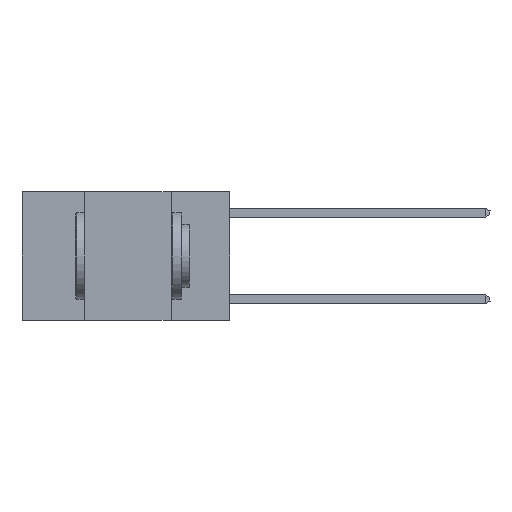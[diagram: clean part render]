
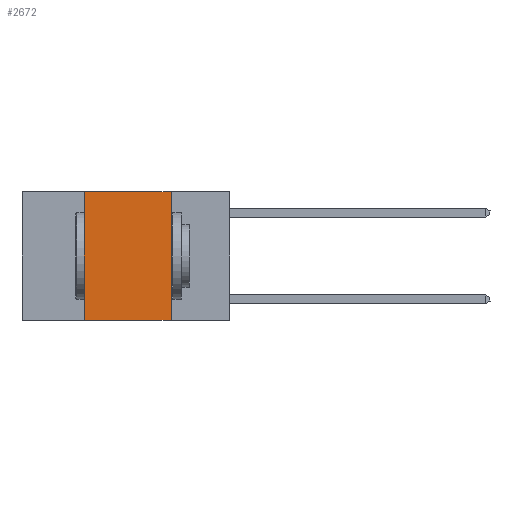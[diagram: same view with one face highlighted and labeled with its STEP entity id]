
A CAD part, left-side view. The second image highlights one B-rep face of the part: STEP entity #2672.
In plain terms, the highlighted planar face has unit normal (-1, 0, 0).
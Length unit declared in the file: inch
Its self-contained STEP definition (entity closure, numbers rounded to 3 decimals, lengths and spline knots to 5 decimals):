
#22 = CARTESIAN_POINT ( 'NONE',  ( 0., 0.6, 0. ) ) ;
#589 = EDGE_LOOP ( 'NONE', ( #2381, #4205, #6792, #6455 ) ) ;
#1487 = CARTESIAN_POINT ( 'NONE',  ( 0., 0.6, -0.37 ) ) ;
#2381 = ORIENTED_EDGE ( 'NONE', *, *, #10137, .F. ) ;
#2543 = CARTESIAN_POINT ( 'NONE',  ( 0., 0.42, 0. ) ) ;
#2587 = EDGE_CURVE ( 'NONE', #9000, #4918, #8205, .T. ) ;
#2672 = ADVANCED_FACE ( 'NONE', ( #7817 ), #2712, .F. ) ;
#2712 = PLANE ( 'NONE',  #8276 ) ;
#3847 = LINE ( 'NONE', #4020, #10657 ) ;
#3904 = VERTEX_POINT ( 'NONE', #10523 ) ;
#3906 = DIRECTION ( 'NONE',  ( 0., 0., -1. ) ) ;
#3972 = CARTESIAN_POINT ( 'NONE',  ( 0., 0.42, 0. ) ) ;
#4020 = CARTESIAN_POINT ( 'NONE',  ( 0., 0.17, 0. ) ) ;
#4205 = ORIENTED_EDGE ( 'NONE', *, *, #8605, .F. ) ;
#4883 = DIRECTION ( 'NONE',  ( 0., -1., 0. ) ) ;
#4918 = VERTEX_POINT ( 'NONE', #6489 ) ;
#5078 = DIRECTION ( 'NONE',  ( 0., -1., 0. ) ) ;
#5554 = VERTEX_POINT ( 'NONE', #2543 ) ;
#5875 = LINE ( 'NONE', #3972, #8883 ) ;
#5887 = VECTOR ( 'NONE', #5078, 39.37008 ) ;
#5988 = DIRECTION ( 'NONE',  ( 0., 0., -1. ) ) ;
#6455 = ORIENTED_EDGE ( 'NONE', *, *, #2587, .T. ) ;
#6489 = CARTESIAN_POINT ( 'NONE',  ( 0., 0.17, -0.37 ) ) ;
#6606 = EDGE_CURVE ( 'NONE', #9000, #5554, #5875, .T. ) ;
#6792 = ORIENTED_EDGE ( 'NONE', *, *, #6606, .F. ) ;
#7817 = FACE_OUTER_BOUND ( 'NONE', #589, .T. ) ;
#8205 = LINE ( 'NONE', #1487, #9547 ) ;
#8276 = AXIS2_PLACEMENT_3D ( 'NONE', #22, #8427, #5988 ) ;
#8427 = DIRECTION ( 'NONE',  ( 1., 0., 0. ) ) ;
#8605 = EDGE_CURVE ( 'NONE', #5554, #3904, #8682, .T. ) ;
#8633 = CARTESIAN_POINT ( 'NONE',  ( 0., 0.42, -0.37 ) ) ;
#8682 = LINE ( 'NONE', #9422, #5887 ) ;
#8883 = VECTOR ( 'NONE', #10012, 39.37008 ) ;
#9000 = VERTEX_POINT ( 'NONE', #8633 ) ;
#9422 = CARTESIAN_POINT ( 'NONE',  ( 0., 0.6, 0. ) ) ;
#9547 = VECTOR ( 'NONE', #4883, 39.37008 ) ;
#10012 = DIRECTION ( 'NONE',  ( 0., 0., 1. ) ) ;
#10137 = EDGE_CURVE ( 'NONE', #3904, #4918, #3847, .T. ) ;
#10523 = CARTESIAN_POINT ( 'NONE',  ( 0., 0.17, 0. ) ) ;
#10657 = VECTOR ( 'NONE', #3906, 39.37008 ) ;
